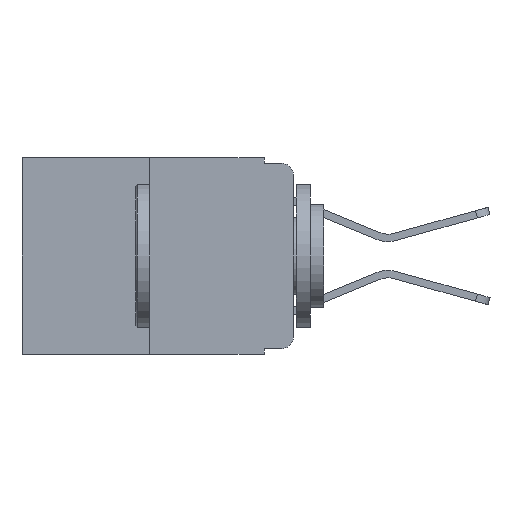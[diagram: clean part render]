
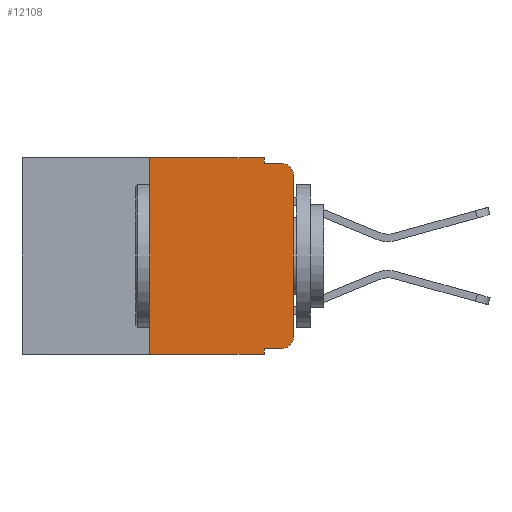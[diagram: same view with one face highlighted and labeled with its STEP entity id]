
A CAD part, left-side view. The second image highlights one B-rep face of the part: STEP entity #12108.
In plain terms, the highlighted planar face has unit normal (-1, 0, 0).
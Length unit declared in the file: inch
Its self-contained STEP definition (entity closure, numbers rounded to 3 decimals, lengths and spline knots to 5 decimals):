
#380 = CIRCLE ( 'NONE', #20931, 0.02 ) ;
#487 = CIRCLE ( 'NONE', #10200, 0.02 ) ;
#673 = EDGE_CURVE ( 'NONE', #4037, #23855, #10303, .T. ) ;
#1037 = ORIENTED_EDGE ( 'NONE', *, *, #16461, .T. ) ;
#1257 = CARTESIAN_POINT ( 'NONE',  ( 0., 0.051, -0.333 ) ) ;
#1515 = EDGE_CURVE ( 'NONE', #20150, #20274, #23734, .T. ) ;
#1657 = VECTOR ( 'NONE', #20798, 39.37008 ) ;
#2475 = ORIENTED_EDGE ( 'NONE', *, *, #24448, .F. ) ;
#2746 = CARTESIAN_POINT ( 'NONE',  ( 0., 0.25, 0. ) ) ;
#3012 = ORIENTED_EDGE ( 'NONE', *, *, #8404, .F. ) ;
#3534 = AXIS2_PLACEMENT_3D ( 'NONE', #22357, #4709, #22450 ) ;
#3605 = VECTOR ( 'NONE', #6861, 39.37008 ) ;
#3983 = EDGE_CURVE ( 'NONE', #23085, #23098, #15270, .T. ) ;
#4023 = EDGE_CURVE ( 'NONE', #23855, #24110, #487, .T. ) ;
#4037 = VERTEX_POINT ( 'NONE', #1257 ) ;
#4554 = CARTESIAN_POINT ( 'NONE',  ( 0., 0.051, -0.333 ) ) ;
#4643 = DIRECTION ( 'NONE',  ( 0., -1., 0. ) ) ;
#4709 = DIRECTION ( 'NONE',  ( 1., 0., 0. ) ) ;
#4951 = ORIENTED_EDGE ( 'NONE', *, *, #22341, .T. ) ;
#5076 = CARTESIAN_POINT ( 'NONE',  ( 0., 0.02, -0.313 ) ) ;
#5335 = LINE ( 'NONE', #23151, #24725 ) ;
#6165 = LINE ( 'NONE', #2746, #22814 ) ;
#6349 = EDGE_CURVE ( 'NONE', #23098, #13590, #5335, .T. ) ;
#6861 = DIRECTION ( 'NONE',  ( 0., 0., -1. ) ) ;
#6886 = DIRECTION ( 'NONE',  ( 0., 0., 1. ) ) ;
#7199 = CARTESIAN_POINT ( 'NONE',  ( 0., 0., 0. ) ) ;
#7341 = CARTESIAN_POINT ( 'NONE',  ( 0., 0.051, 0. ) ) ;
#8060 = CARTESIAN_POINT ( 'NONE',  ( 0., 0.25, 0. ) ) ;
#8271 = DIRECTION ( 'NONE',  ( -1., 0., 0. ) ) ;
#8404 = EDGE_CURVE ( 'NONE', #4037, #20274, #22322, .T. ) ;
#8693 = CARTESIAN_POINT ( 'NONE',  ( 0., 0.02, -0.333 ) ) ;
#9277 = EDGE_CURVE ( 'NONE', #11758, #23085, #19497, .T. ) ;
#9519 = DIRECTION ( 'NONE',  ( 0., -1., 0. ) ) ;
#9775 = ORIENTED_EDGE ( 'NONE', *, *, #3983, .F. ) ;
#10200 = AXIS2_PLACEMENT_3D ( 'NONE', #5076, #12944, #16832 ) ;
#10303 = LINE ( 'NONE', #4554, #16135 ) ;
#10325 = CARTESIAN_POINT ( 'NONE',  ( 0., 0.02, -0.03 ) ) ;
#10419 = ORIENTED_EDGE ( 'NONE', *, *, #1515, .T. ) ;
#10703 = PLANE ( 'NONE',  #3534 ) ;
#11758 = VERTEX_POINT ( 'NONE', #8060 ) ;
#12108 = ADVANCED_FACE ( 'NONE', ( #23660 ), #10703, .F. ) ;
#12518 = CARTESIAN_POINT ( 'NONE',  ( 0., 0.051, 0. ) ) ;
#12944 = DIRECTION ( 'NONE',  ( -1., 0., 0. ) ) ;
#13002 = VECTOR ( 'NONE', #15095, 39.37008 ) ;
#13590 = VERTEX_POINT ( 'NONE', #24006 ) ;
#13793 = CARTESIAN_POINT ( 'NONE',  ( 0., 0.473, 0. ) ) ;
#14292 = ORIENTED_EDGE ( 'NONE', *, *, #6349, .F. ) ;
#15095 = DIRECTION ( 'NONE',  ( 0., 0., 1. ) ) ;
#15270 = LINE ( 'NONE', #12518, #3605 ) ;
#15803 = ORIENTED_EDGE ( 'NONE', *, *, #9277, .F. ) ;
#16135 = VECTOR ( 'NONE', #4643, 39.37008 ) ;
#16280 = CARTESIAN_POINT ( 'NONE',  ( 0., 0., -0.03 ) ) ;
#16461 = EDGE_CURVE ( 'NONE', #22806, #13590, #380, .T. ) ;
#16832 = DIRECTION ( 'NONE',  ( 0., 0., -1. ) ) ;
#16999 = ORIENTED_EDGE ( 'NONE', *, *, #673, .T. ) ;
#17081 = EDGE_LOOP ( 'NONE', ( #4951, #1037, #14292, #9775, #15803, #2475, #10419, #3012, #16999, #20351 ) ) ;
#17940 = CARTESIAN_POINT ( 'NONE',  ( 0., 0., -0.313 ) ) ;
#18759 = CARTESIAN_POINT ( 'NONE',  ( 0., 0.051, -0.343 ) ) ;
#19181 = DIRECTION ( 'NONE',  ( 0., -1., 0. ) ) ;
#19497 = LINE ( 'NONE', #13793, #20738 ) ;
#19757 = CARTESIAN_POINT ( 'NONE',  ( 0., 0.25, -0.343 ) ) ;
#19989 = DIRECTION ( 'NONE',  ( 0., 0., -1. ) ) ;
#20150 = VERTEX_POINT ( 'NONE', #19757 ) ;
#20274 = VERTEX_POINT ( 'NONE', #18759 ) ;
#20351 = ORIENTED_EDGE ( 'NONE', *, *, #4023, .T. ) ;
#20738 = VECTOR ( 'NONE', #9519, 39.37008 ) ;
#20798 = DIRECTION ( 'NONE',  ( 0., 0., -1. ) ) ;
#20931 = AXIS2_PLACEMENT_3D ( 'NONE', #10325, #8271, #19989 ) ;
#20971 = CARTESIAN_POINT ( 'NONE',  ( 0., 0.051, 0. ) ) ;
#22321 = DIRECTION ( 'NONE',  ( 0., -1., 0. ) ) ;
#22322 = LINE ( 'NONE', #20971, #1657 ) ;
#22341 = EDGE_CURVE ( 'NONE', #24110, #22806, #23829, .T. ) ;
#22357 = CARTESIAN_POINT ( 'NONE',  ( 0., 0.473, 0. ) ) ;
#22450 = DIRECTION ( 'NONE',  ( 0., 0., -1. ) ) ;
#22806 = VERTEX_POINT ( 'NONE', #16280 ) ;
#22814 = VECTOR ( 'NONE', #6886, 39.37008 ) ;
#22827 = VECTOR ( 'NONE', #22321, 39.37008 ) ;
#23085 = VERTEX_POINT ( 'NONE', #7341 ) ;
#23098 = VERTEX_POINT ( 'NONE', #23111 ) ;
#23111 = CARTESIAN_POINT ( 'NONE',  ( 0., 0.051, -0.01 ) ) ;
#23151 = CARTESIAN_POINT ( 'NONE',  ( 0., 0.051, -0.01 ) ) ;
#23660 = FACE_OUTER_BOUND ( 'NONE', #17081, .T. ) ;
#23734 = LINE ( 'NONE', #24290, #22827 ) ;
#23829 = LINE ( 'NONE', #7199, #13002 ) ;
#23855 = VERTEX_POINT ( 'NONE', #8693 ) ;
#24006 = CARTESIAN_POINT ( 'NONE',  ( 0., 0.02, -0.01 ) ) ;
#24110 = VERTEX_POINT ( 'NONE', #17940 ) ;
#24290 = CARTESIAN_POINT ( 'NONE',  ( 0., 0.473, -0.343 ) ) ;
#24448 = EDGE_CURVE ( 'NONE', #20150, #11758, #6165, .T. ) ;
#24725 = VECTOR ( 'NONE', #19181, 39.37008 ) ;
